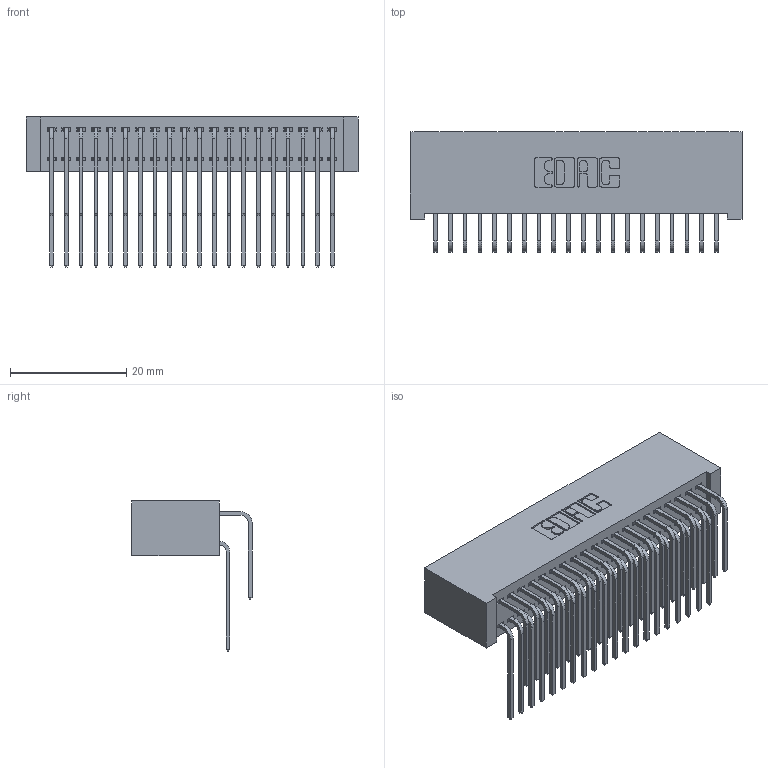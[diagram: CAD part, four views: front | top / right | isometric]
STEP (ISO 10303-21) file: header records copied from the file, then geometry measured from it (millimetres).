
FILE_DESCRIPTION (( 'STEP AP203' ), '1' );
FILE_NAME ('392-040-559-201.STEP', '2019-10-07T20:20:19', ( '' ), ( '' ), 'SwSTEP 2.0', 'SolidWorks 2016', '' );
FILE_SCHEMA (( 'CONFIG_CONTROL_DESIGN' ));
Length unit declared in the file: inch
Products named in the file (4): 345-292-001_559 Tail - 2; 392-040-559-201; 342 Part_Lugless; 345-292-001_558 559 Tail - 1
Assembly tree (41 placements, depth 2):
  392-040-559-201
    342 Part_Lugless
    345-292-001_558 559 Tail - 1  x20
    345-292-001_559 Tail - 2  x20
Bounding box: 57.05 x 20.64 x 25.78 mm (x, y, z)
Volume: 5691.9 mm3; surface area: 10213 mm2
Topology: 41 solids, 41 shells, 2262 faces, 6715 edges, 4422 vertices
Faces by surface type: plane 1582, cylinder 680
Entity records: 17087 total; most frequent: CARTESIAN_POINT 2905, ORIENTED_EDGE 2790, DIRECTION 2495, EDGE_CURVE 1395, VECTOR 1235, LINE 1235, VERTEX_POINT 926, AXIS2_PLACEMENT_3D 630
